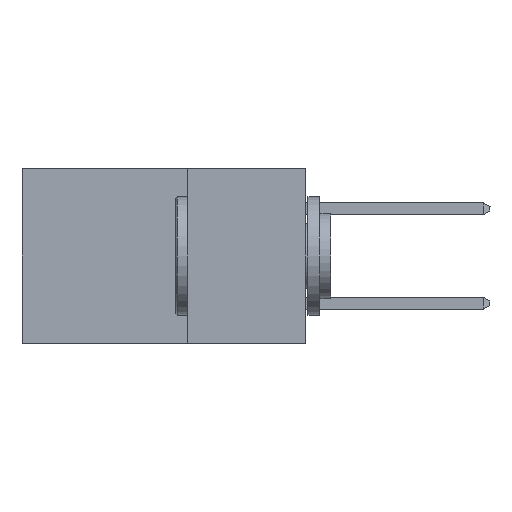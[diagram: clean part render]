
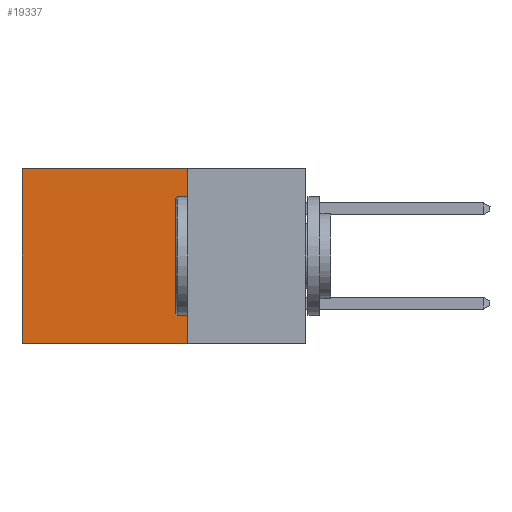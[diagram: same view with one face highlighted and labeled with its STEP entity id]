
A CAD part, left-side view. The second image highlights one B-rep face of the part: STEP entity #19337.
In plain terms, the highlighted planar face has unit normal (-1, 0, 0).
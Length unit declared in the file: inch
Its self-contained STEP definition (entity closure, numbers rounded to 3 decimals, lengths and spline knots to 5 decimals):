
#620 = VERTEX_POINT ( 'NONE', #5166 ) ;
#839 = ORIENTED_EDGE ( 'NONE', *, *, #17179, .F. ) ;
#2461 = VECTOR ( 'NONE', #8027, 39.37008 ) ;
#3095 = CARTESIAN_POINT ( 'NONE',  ( 0.298, 0.6, 0. ) ) ;
#3900 = ORIENTED_EDGE ( 'NONE', *, *, #9944, .F. ) ;
#5166 = CARTESIAN_POINT ( 'NONE',  ( 0.298, 0.25, 0. ) ) ;
#5940 = LINE ( 'NONE', #3095, #2461 ) ;
#6146 = LINE ( 'NONE', #29312, #16939 ) ;
#8027 = DIRECTION ( 'NONE',  ( 0., 0., -1. ) ) ;
#9477 = ORIENTED_EDGE ( 'NONE', *, *, #13685, .T. ) ;
#9859 = VERTEX_POINT ( 'NONE', #20042 ) ;
#9944 = EDGE_CURVE ( 'NONE', #16912, #13149, #22885, .T. ) ;
#10431 = EDGE_LOOP ( 'NONE', ( #9477, #3900, #839, #20710 ) ) ;
#10803 = CARTESIAN_POINT ( 'NONE',  ( 0.298, 0.25, -0.37 ) ) ;
#12138 = DIRECTION ( 'NONE',  ( 1., 0., 0. ) ) ;
#13149 = VERTEX_POINT ( 'NONE', #26200 ) ;
#13685 = EDGE_CURVE ( 'NONE', #9859, #13149, #5940, .T. ) ;
#14224 = DIRECTION ( 'NONE',  ( 0., 1., 0. ) ) ;
#15597 = VECTOR ( 'NONE', #14224, 39.37008 ) ;
#15650 = EDGE_CURVE ( 'NONE', #620, #9859, #30129, .T. ) ;
#16912 = VERTEX_POINT ( 'NONE', #10803 ) ;
#16939 = VECTOR ( 'NONE', #31791, 39.37008 ) ;
#17179 = EDGE_CURVE ( 'NONE', #620, #16912, #6146, .T. ) ;
#19337 = ADVANCED_FACE ( 'NONE', ( #27806 ), #19556, .F. ) ;
#19556 = PLANE ( 'NONE',  #27091 ) ;
#20042 = CARTESIAN_POINT ( 'NONE',  ( 0.298, 0.6, 0. ) ) ;
#20415 = CARTESIAN_POINT ( 'NONE',  ( 0.298, 0.25, 0. ) ) ;
#20710 = ORIENTED_EDGE ( 'NONE', *, *, #15650, .T. ) ;
#21616 = VECTOR ( 'NONE', #27353, 39.37008 ) ;
#22885 = LINE ( 'NONE', #26683, #15597 ) ;
#26200 = CARTESIAN_POINT ( 'NONE',  ( 0.298, 0.6, -0.37 ) ) ;
#26683 = CARTESIAN_POINT ( 'NONE',  ( 0.298, 0.25, -0.37 ) ) ;
#26981 = DIRECTION ( 'NONE',  ( 0., 0., -1. ) ) ;
#27091 = AXIS2_PLACEMENT_3D ( 'NONE', #20415, #12138, #26981 ) ;
#27353 = DIRECTION ( 'NONE',  ( 0., 1., 0. ) ) ;
#27806 = FACE_OUTER_BOUND ( 'NONE', #10431, .T. ) ;
#29312 = CARTESIAN_POINT ( 'NONE',  ( 0.298, 0.25, 0. ) ) ;
#29756 = CARTESIAN_POINT ( 'NONE',  ( 0.298, 0.25, 0. ) ) ;
#30129 = LINE ( 'NONE', #29756, #21616 ) ;
#31791 = DIRECTION ( 'NONE',  ( 0., 0., -1. ) ) ;
